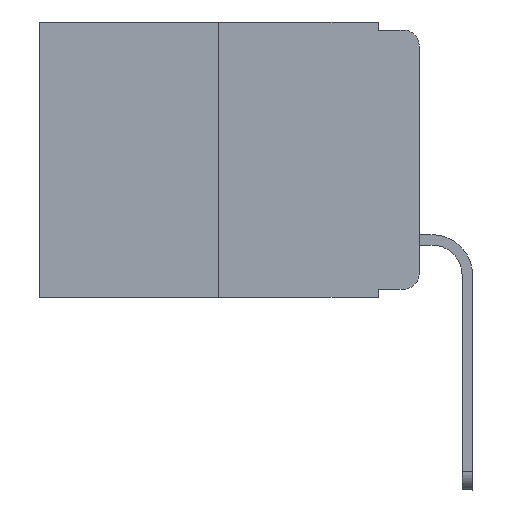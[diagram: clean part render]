
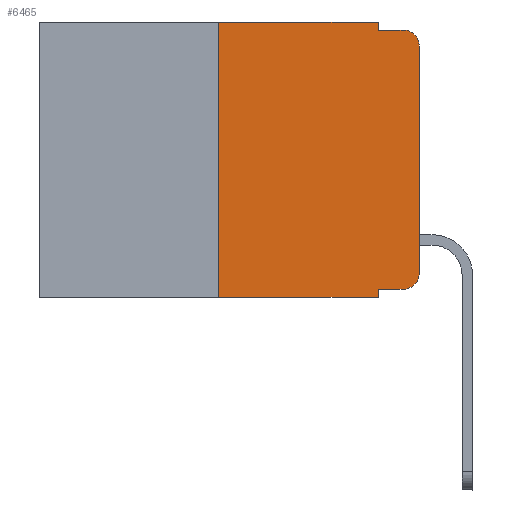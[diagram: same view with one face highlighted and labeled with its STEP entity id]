
A CAD part, left-side view. The second image highlights one B-rep face of the part: STEP entity #6465.
In plain terms, the highlighted planar face has unit normal (-1, 0, 0).
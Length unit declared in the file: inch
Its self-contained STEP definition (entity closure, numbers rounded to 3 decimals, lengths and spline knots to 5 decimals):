
#311 = DIRECTION ( 'NONE',  ( 0., 0., -1. ) ) ;
#441 = DIRECTION ( 'NONE',  ( 0., 0., 1. ) ) ;
#1044 = VECTOR ( 'NONE', #13132, 39.37008 ) ;
#1315 = ORIENTED_EDGE ( 'NONE', *, *, #17476, .T. ) ;
#1538 = CARTESIAN_POINT ( 'NONE',  ( 0., 0.051, -0.333 ) ) ;
#1621 = DIRECTION ( 'NONE',  ( 0., 0., -1. ) ) ;
#1779 = EDGE_LOOP ( 'NONE', ( #22913, #18307, #16169, #11295, #5338, #7903, #1315, #21910, #5873, #17780 ) ) ;
#1983 = EDGE_CURVE ( 'NONE', #20277, #3605, #13395, .T. ) ;
#3605 = VERTEX_POINT ( 'NONE', #10001 ) ;
#3754 = DIRECTION ( 'NONE',  ( -1., 0., 0. ) ) ;
#4106 = AXIS2_PLACEMENT_3D ( 'NONE', #6114, #9272, #311 ) ;
#4704 = VERTEX_POINT ( 'NONE', #5895 ) ;
#5338 = ORIENTED_EDGE ( 'NONE', *, *, #14301, .F. ) ;
#5510 = CARTESIAN_POINT ( 'NONE',  ( 0., 0.02, -0.313 ) ) ;
#5697 = CARTESIAN_POINT ( 'NONE',  ( 0., 0., -0.03 ) ) ;
#5873 = ORIENTED_EDGE ( 'NONE', *, *, #17349, .T. ) ;
#5895 = CARTESIAN_POINT ( 'NONE',  ( 0., 0.051, 0. ) ) ;
#6001 = VERTEX_POINT ( 'NONE', #5697 ) ;
#6114 = CARTESIAN_POINT ( 'NONE',  ( 0., 0.473, 0. ) ) ;
#6241 = EDGE_CURVE ( 'NONE', #4704, #19395, #19347, .T. ) ;
#6465 = ADVANCED_FACE ( 'NONE', ( #12816 ), #22035, .F. ) ;
#6781 = LINE ( 'NONE', #15713, #13029 ) ;
#6964 = CARTESIAN_POINT ( 'NONE',  ( 0., 0.02, -0.03 ) ) ;
#7069 = VECTOR ( 'NONE', #8471, 39.37008 ) ;
#7432 = CARTESIAN_POINT ( 'NONE',  ( 0., 0.051, -0.01 ) ) ;
#7781 = VECTOR ( 'NONE', #16001, 39.37008 ) ;
#7903 = ORIENTED_EDGE ( 'NONE', *, *, #1983, .F. ) ;
#8351 = VERTEX_POINT ( 'NONE', #9007 ) ;
#8414 = DIRECTION ( 'NONE',  ( 0., -1., 0. ) ) ;
#8471 = DIRECTION ( 'NONE',  ( 0., 0., -1. ) ) ;
#8475 = LINE ( 'NONE', #15645, #13333 ) ;
#8964 = CARTESIAN_POINT ( 'NONE',  ( 0., 0.02, -0.333 ) ) ;
#9007 = CARTESIAN_POINT ( 'NONE',  ( 0., 0., -0.313 ) ) ;
#9253 = DIRECTION ( 'NONE',  ( 0., -1., 0. ) ) ;
#9272 = DIRECTION ( 'NONE',  ( 1., 0., 0. ) ) ;
#9386 = LINE ( 'NONE', #14667, #17167 ) ;
#10001 = CARTESIAN_POINT ( 'NONE',  ( 0., 0.25, 0. ) ) ;
#10347 = EDGE_CURVE ( 'NONE', #14082, #18042, #17536, .T. ) ;
#10607 = CARTESIAN_POINT ( 'NONE',  ( 0., 0.473, 0. ) ) ;
#10926 = DIRECTION ( 'NONE',  ( 0., 0., -1. ) ) ;
#10947 = LINE ( 'NONE', #10607, #7781 ) ;
#11207 = EDGE_CURVE ( 'NONE', #6001, #16468, #18322, .T. ) ;
#11295 = ORIENTED_EDGE ( 'NONE', *, *, #6241, .F. ) ;
#11350 = VECTOR ( 'NONE', #441, 39.37008 ) ;
#12137 = DIRECTION ( 'NONE',  ( 0., -1., 0. ) ) ;
#12680 = AXIS2_PLACEMENT_3D ( 'NONE', #6964, #14275, #14145 ) ;
#12816 = FACE_OUTER_BOUND ( 'NONE', #1779, .T. ) ;
#12868 = VERTEX_POINT ( 'NONE', #8964 ) ;
#13029 = VECTOR ( 'NONE', #8414, 39.37008 ) ;
#13051 = AXIS2_PLACEMENT_3D ( 'NONE', #5510, #3754, #1621 ) ;
#13132 = DIRECTION ( 'NONE',  ( 0., 0., 1. ) ) ;
#13333 = VECTOR ( 'NONE', #12137, 39.37008 ) ;
#13395 = LINE ( 'NONE', #15267, #11350 ) ;
#13893 = CARTESIAN_POINT ( 'NONE',  ( 0., 0.051, 0. ) ) ;
#13920 = CARTESIAN_POINT ( 'NONE',  ( 0., 0.051, -0.343 ) ) ;
#14082 = VERTEX_POINT ( 'NONE', #1538 ) ;
#14145 = DIRECTION ( 'NONE',  ( 0., 0., -1. ) ) ;
#14275 = DIRECTION ( 'NONE',  ( -1., 0., 0. ) ) ;
#14301 = EDGE_CURVE ( 'NONE', #3605, #4704, #10947, .T. ) ;
#14445 = CARTESIAN_POINT ( 'NONE',  ( 0., 0.051, 0. ) ) ;
#14654 = CARTESIAN_POINT ( 'NONE',  ( 0., 0., 0. ) ) ;
#14667 = CARTESIAN_POINT ( 'NONE',  ( 0., 0.051, -0.333 ) ) ;
#14672 = EDGE_CURVE ( 'NONE', #12868, #8351, #23265, .T. ) ;
#15249 = EDGE_CURVE ( 'NONE', #8351, #6001, #16544, .T. ) ;
#15267 = CARTESIAN_POINT ( 'NONE',  ( 0., 0.25, 0. ) ) ;
#15645 = CARTESIAN_POINT ( 'NONE',  ( 0., 0.051, -0.01 ) ) ;
#15713 = CARTESIAN_POINT ( 'NONE',  ( 0., 0.473, -0.343 ) ) ;
#16001 = DIRECTION ( 'NONE',  ( 0., -1., 0. ) ) ;
#16169 = ORIENTED_EDGE ( 'NONE', *, *, #18472, .F. ) ;
#16468 = VERTEX_POINT ( 'NONE', #21278 ) ;
#16517 = VECTOR ( 'NONE', #10926, 39.37008 ) ;
#16544 = LINE ( 'NONE', #14654, #1044 ) ;
#17167 = VECTOR ( 'NONE', #9253, 39.37008 ) ;
#17349 = EDGE_CURVE ( 'NONE', #14082, #12868, #9386, .T. ) ;
#17476 = EDGE_CURVE ( 'NONE', #20277, #18042, #6781, .T. ) ;
#17536 = LINE ( 'NONE', #13893, #7069 ) ;
#17780 = ORIENTED_EDGE ( 'NONE', *, *, #14672, .T. ) ;
#17802 = CARTESIAN_POINT ( 'NONE',  ( 0., 0.25, -0.343 ) ) ;
#18042 = VERTEX_POINT ( 'NONE', #13920 ) ;
#18307 = ORIENTED_EDGE ( 'NONE', *, *, #11207, .T. ) ;
#18322 = CIRCLE ( 'NONE', #12680, 0.02 ) ;
#18472 = EDGE_CURVE ( 'NONE', #19395, #16468, #8475, .T. ) ;
#19347 = LINE ( 'NONE', #14445, #16517 ) ;
#19395 = VERTEX_POINT ( 'NONE', #7432 ) ;
#20277 = VERTEX_POINT ( 'NONE', #17802 ) ;
#21278 = CARTESIAN_POINT ( 'NONE',  ( 0., 0.02, -0.01 ) ) ;
#21910 = ORIENTED_EDGE ( 'NONE', *, *, #10347, .F. ) ;
#22035 = PLANE ( 'NONE',  #4106 ) ;
#22913 = ORIENTED_EDGE ( 'NONE', *, *, #15249, .T. ) ;
#23265 = CIRCLE ( 'NONE', #13051, 0.02 ) ;
